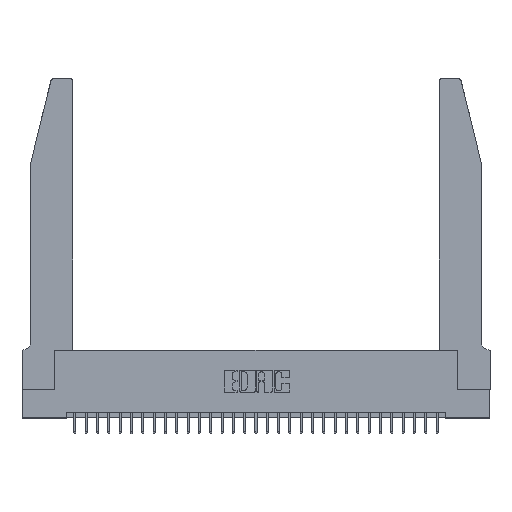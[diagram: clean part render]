
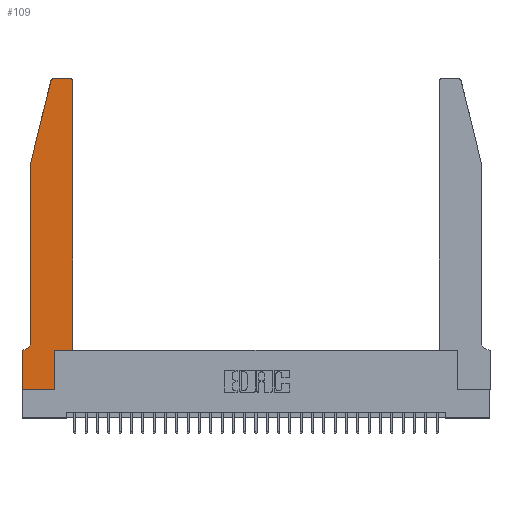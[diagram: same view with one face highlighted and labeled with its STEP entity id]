
A CAD part, top view. The second image highlights one B-rep face of the part: STEP entity #109.
In plain terms, the highlighted planar face has unit normal (0, 0, 1).
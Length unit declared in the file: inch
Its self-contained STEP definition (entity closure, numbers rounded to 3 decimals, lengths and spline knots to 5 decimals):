
#54 = CARTESIAN_POINT ( 'NONE',  ( 0., 0.35, 0.37 ) ) ;
#89 = CIRCLE ( 'NONE', #27994, 0.07 ) ;
#109 = ADVANCED_FACE ( 'NONE', ( #9682 ), #29422, .T. ) ;
#142 = VERTEX_POINT ( 'NONE', #20036 ) ;
#274 = DIRECTION ( 'NONE',  ( -0.239, -0.971, 0. ) ) ;
#315 = EDGE_CURVE ( 'NONE', #23861, #31310, #8856, .T. ) ;
#676 = VECTOR ( 'NONE', #13655, 39.37008 ) ;
#902 = VERTEX_POINT ( 'NONE', #15422 ) ;
#907 = CARTESIAN_POINT ( 'NONE',  ( 0., 0., 0.37 ) ) ;
#2279 = AXIS2_PLACEMENT_3D ( 'NONE', #21120, #6719, #21275 ) ;
#2942 = CARTESIAN_POINT ( 'NONE',  ( 0.2865, 0.35, 0.37 ) ) ;
#3041 = ORIENTED_EDGE ( 'NONE', *, *, #25282, .T. ) ;
#3083 = VERTEX_POINT ( 'NONE', #54 ) ;
#3117 = EDGE_CURVE ( 'NONE', #24566, #23861, #24482, .T. ) ;
#3254 = DIRECTION ( 'NONE',  ( -1., 0., 0. ) ) ;
#3539 = EDGE_CURVE ( 'NONE', #12622, #3083, #15041, .T. ) ;
#3632 = EDGE_CURVE ( 'NONE', #31310, #902, #27998, .T. ) ;
#3729 = CARTESIAN_POINT ( 'NONE',  ( 0.25487, 2.72718, 0.37 ) ) ;
#5530 = CARTESIAN_POINT ( 'NONE',  ( 0.2865, 0., 0.37 ) ) ;
#5648 = CARTESIAN_POINT ( 'NONE',  ( 0., 0.35, 0.37 ) ) ;
#5741 = AXIS2_PLACEMENT_3D ( 'NONE', #5648, #25706, #20190 ) ;
#5759 = CARTESIAN_POINT ( 'NONE',  ( 0.0755, 2., 0.37 ) ) ;
#5813 = EDGE_CURVE ( 'NONE', #21022, #25337, #9509, .T. ) ;
#6719 = DIRECTION ( 'NONE',  ( 0., 0., 1. ) ) ;
#6784 = EDGE_CURVE ( 'NONE', #29099, #9796, #29555, .T. ) ;
#7292 = DIRECTION ( 'NONE',  ( -1., 0., 0. ) ) ;
#8123 = LINE ( 'NONE', #27866, #22191 ) ;
#8856 = LINE ( 'NONE', #13865, #28991 ) ;
#9031 = EDGE_CURVE ( 'NONE', #11187, #21022, #8123, .T. ) ;
#9036 = VECTOR ( 'NONE', #9654, 39.37008 ) ;
#9509 = CIRCLE ( 'NONE', #2279, 0.03 ) ;
#9603 = CARTESIAN_POINT ( 'NONE',  ( 0., 0., 0.37 ) ) ;
#9654 = DIRECTION ( 'NONE',  ( 0., -1., 0. ) ) ;
#9682 = FACE_OUTER_BOUND ( 'NONE', #14405, .T. ) ;
#9796 = VERTEX_POINT ( 'NONE', #25518 ) ;
#9837 = EDGE_CURVE ( 'NONE', #25337, #29099, #25194, .T. ) ;
#9974 = CARTESIAN_POINT ( 'NONE',  ( 0.0755, 2., 0.37 ) ) ;
#10358 = ORIENTED_EDGE ( 'NONE', *, *, #13337, .T. ) ;
#10863 = DIRECTION ( 'NONE',  ( 1., 0., 0. ) ) ;
#11144 = ORIENTED_EDGE ( 'NONE', *, *, #28031, .T. ) ;
#11187 = VERTEX_POINT ( 'NONE', #11412 ) ;
#11412 = CARTESIAN_POINT ( 'NONE',  ( 0.4205, 2.75, 0.37 ) ) ;
#11484 = DIRECTION ( 'NONE',  ( 0., 0., 1. ) ) ;
#12622 = VERTEX_POINT ( 'NONE', #31204 ) ;
#13337 = EDGE_CURVE ( 'NONE', #142, #11187, #31697, .T. ) ;
#13464 = ORIENTED_EDGE ( 'NONE', *, *, #3539, .T. ) ;
#13655 = DIRECTION ( 'NONE',  ( 0., -1., 0. ) ) ;
#13865 = CARTESIAN_POINT ( 'NONE',  ( 0.2865, 0.35, 0.37 ) ) ;
#14405 = EDGE_LOOP ( 'NONE', ( #31099, #16006, #26317, #23849, #3041, #13464, #11144, #24795, #25165, #18136, #18594, #10358 ) ) ;
#15041 = LINE ( 'NONE', #19422, #17246 ) ;
#15422 = CARTESIAN_POINT ( 'NONE',  ( 0.4505, 0.35, 0.37 ) ) ;
#15871 = CARTESIAN_POINT ( 'NONE',  ( 0.0055, 0.42, 0.37 ) ) ;
#16006 = ORIENTED_EDGE ( 'NONE', *, *, #5813, .T. ) ;
#17246 = VECTOR ( 'NONE', #7292, 39.37008 ) ;
#17538 = CARTESIAN_POINT ( 'NONE',  ( 0., 0., 0.37 ) ) ;
#18136 = ORIENTED_EDGE ( 'NONE', *, *, #3632, .T. ) ;
#18594 = ORIENTED_EDGE ( 'NONE', *, *, #28358, .T. ) ;
#18746 = AXIS2_PLACEMENT_3D ( 'NONE', #26244, #11484, #10863 ) ;
#19422 = CARTESIAN_POINT ( 'NONE',  ( 0.0755, 0.35, 0.37 ) ) ;
#19835 = CARTESIAN_POINT ( 'NONE',  ( 0.0755, 2., 0.37 ) ) ;
#20036 = CARTESIAN_POINT ( 'NONE',  ( 0.4505, 2.72, 0.37 ) ) ;
#20190 = DIRECTION ( 'NONE',  ( 1., 0., 0. ) ) ;
#20440 = CARTESIAN_POINT ( 'NONE',  ( 0.4505, 0.35, 0.37 ) ) ;
#20905 = DIRECTION ( 'NONE',  ( 0., 1., 0. ) ) ;
#21022 = VERTEX_POINT ( 'NONE', #25805 ) ;
#21120 = CARTESIAN_POINT ( 'NONE',  ( 0.284, 2.72, 0.37 ) ) ;
#21275 = DIRECTION ( 'NONE',  ( 1., 0., 0. ) ) ;
#21609 = VECTOR ( 'NONE', #274, 39.37008 ) ;
#21864 = VECTOR ( 'NONE', #20905, 39.37008 ) ;
#22056 = DIRECTION ( 'NONE',  ( 1., 0., 0. ) ) ;
#22191 = VECTOR ( 'NONE', #25766, 39.37008 ) ;
#22397 = VECTOR ( 'NONE', #25420, 39.37008 ) ;
#23062 = LINE ( 'NONE', #907, #676 ) ;
#23849 = ORIENTED_EDGE ( 'NONE', *, *, #6784, .T. ) ;
#23861 = VERTEX_POINT ( 'NONE', #5530 ) ;
#24482 = LINE ( 'NONE', #9603, #29629 ) ;
#24566 = VERTEX_POINT ( 'NONE', #17538 ) ;
#24795 = ORIENTED_EDGE ( 'NONE', *, *, #3117, .T. ) ;
#25165 = ORIENTED_EDGE ( 'NONE', *, *, #315, .T. ) ;
#25194 = LINE ( 'NONE', #9974, #21609 ) ;
#25282 = EDGE_CURVE ( 'NONE', #9796, #12622, #89, .T. ) ;
#25337 = VERTEX_POINT ( 'NONE', #3729 ) ;
#25420 = DIRECTION ( 'NONE',  ( 1., 0., 0. ) ) ;
#25518 = CARTESIAN_POINT ( 'NONE',  ( 0.0755, 0.42, 0.37 ) ) ;
#25706 = DIRECTION ( 'NONE',  ( 0., 0., 1. ) ) ;
#25761 = DIRECTION ( 'NONE',  ( 0., 0., -1. ) ) ;
#25766 = DIRECTION ( 'NONE',  ( -1., 0., 0. ) ) ;
#25786 = LINE ( 'NONE', #20440, #21864 ) ;
#25805 = CARTESIAN_POINT ( 'NONE',  ( 0.284, 2.75, 0.37 ) ) ;
#26244 = CARTESIAN_POINT ( 'NONE',  ( 0.4205, 2.72, 0.37 ) ) ;
#26317 = ORIENTED_EDGE ( 'NONE', *, *, #9837, .T. ) ;
#26338 = DIRECTION ( 'NONE',  ( 0., 1., 0. ) ) ;
#27866 = CARTESIAN_POINT ( 'NONE',  ( 0.2605, 2.75, 0.37 ) ) ;
#27994 = AXIS2_PLACEMENT_3D ( 'NONE', #15871, #25761, #3254 ) ;
#27998 = LINE ( 'NONE', #28158, #22397 ) ;
#28031 = EDGE_CURVE ( 'NONE', #3083, #24566, #23062, .T. ) ;
#28158 = CARTESIAN_POINT ( 'NONE',  ( 0.4505, 0.35, 0.37 ) ) ;
#28358 = EDGE_CURVE ( 'NONE', #902, #142, #25786, .T. ) ;
#28991 = VECTOR ( 'NONE', #26338, 39.37008 ) ;
#29099 = VERTEX_POINT ( 'NONE', #5759 ) ;
#29422 = PLANE ( 'NONE',  #5741 ) ;
#29555 = LINE ( 'NONE', #19835, #9036 ) ;
#29629 = VECTOR ( 'NONE', #22056, 39.37008 ) ;
#31099 = ORIENTED_EDGE ( 'NONE', *, *, #9031, .T. ) ;
#31204 = CARTESIAN_POINT ( 'NONE',  ( 0.0055, 0.35, 0.37 ) ) ;
#31310 = VERTEX_POINT ( 'NONE', #2942 ) ;
#31697 = CIRCLE ( 'NONE', #18746, 0.03 ) ;
